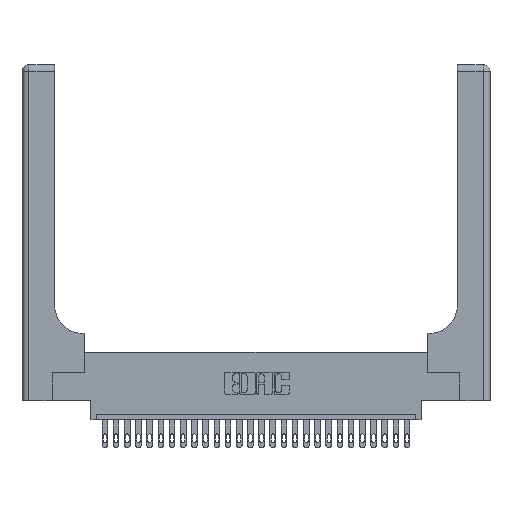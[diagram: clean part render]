
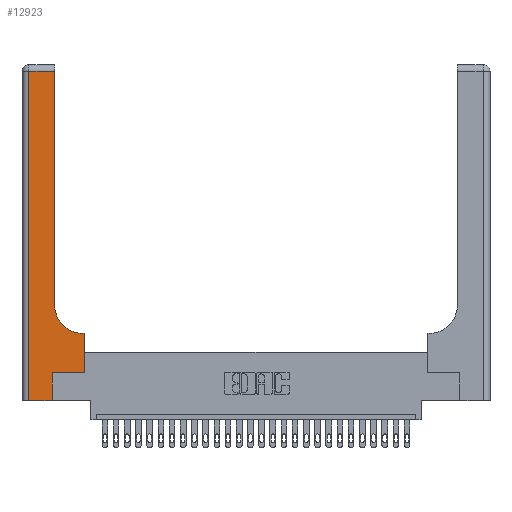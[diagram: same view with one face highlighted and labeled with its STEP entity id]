
A CAD part, top view. The second image highlights one B-rep face of the part: STEP entity #12923.
In plain terms, the highlighted planar face has unit normal (0, 0, 1).
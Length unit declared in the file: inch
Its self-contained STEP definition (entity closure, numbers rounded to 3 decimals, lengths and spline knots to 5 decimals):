
#1087 = VERTEX_POINT ( 'NONE', #15243 ) ;
#1124 = EDGE_CURVE ( 'NONE', #19941, #24948, #12231, .T. ) ;
#1284 = EDGE_CURVE ( 'NONE', #19862, #2779, #8533, .T. ) ;
#1878 = CARTESIAN_POINT ( 'NONE',  ( 0.06, 0., 0.37 ) ) ;
#2245 = CARTESIAN_POINT ( 'NONE',  ( 0.5585, 0.25, 0.37 ) ) ;
#2260 = EDGE_LOOP ( 'NONE', ( #27767, #25125, #16244, #16059, #4777, #15587, #26171, #25153, #7526 ) ) ;
#2608 = EDGE_CURVE ( 'NONE', #4192, #10452, #23671, .T. ) ;
#2779 = VERTEX_POINT ( 'NONE', #12306 ) ;
#2993 = CARTESIAN_POINT ( 'NONE',  ( 0.5415, 0.6, 0.37 ) ) ;
#3927 = CARTESIAN_POINT ( 'NONE',  ( 0.06, 2.94, 0.37 ) ) ;
#4192 = VERTEX_POINT ( 'NONE', #7046 ) ;
#4509 = DIRECTION ( 'NONE',  ( 1., 0., 0. ) ) ;
#4777 = ORIENTED_EDGE ( 'NONE', *, *, #21290, .T. ) ;
#5163 = VECTOR ( 'NONE', #21841, 39.37008 ) ;
#6279 = CARTESIAN_POINT ( 'NONE',  ( 0.2915, 0.85, 0.37 ) ) ;
#6753 = VERTEX_POINT ( 'NONE', #3927 ) ;
#7046 = CARTESIAN_POINT ( 'NONE',  ( 0.5585, 0.6, 0.37 ) ) ;
#7117 = CARTESIAN_POINT ( 'NONE',  ( 0.06, 3., 0.37 ) ) ;
#7526 = ORIENTED_EDGE ( 'NONE', *, *, #10643, .T. ) ;
#8276 = DIRECTION ( 'NONE',  ( -1., 0., 0. ) ) ;
#8343 = CARTESIAN_POINT ( 'NONE',  ( 0., 3., 0.37 ) ) ;
#8533 = LINE ( 'NONE', #26169, #28185 ) ;
#9710 = FACE_OUTER_BOUND ( 'NONE', #2260, .T. ) ;
#10094 = EDGE_CURVE ( 'NONE', #2779, #6753, #20398, .T. ) ;
#10138 = CARTESIAN_POINT ( 'NONE',  ( 0.5585, 0.25, 0.37 ) ) ;
#10452 = VERTEX_POINT ( 'NONE', #2993 ) ;
#10643 = EDGE_CURVE ( 'NONE', #10452, #19862, #11910, .T. ) ;
#10794 = DIRECTION ( 'NONE',  ( 0., 0., -1. ) ) ;
#11910 = CIRCLE ( 'NONE', #17909, 0.25 ) ;
#12019 = EDGE_CURVE ( 'NONE', #24948, #4192, #18613, .T. ) ;
#12231 = LINE ( 'NONE', #18712, #26135 ) ;
#12306 = CARTESIAN_POINT ( 'NONE',  ( 0.2915, 2.94, 0.37 ) ) ;
#12521 = DIRECTION ( 'NONE',  ( 0., 1., 0. ) ) ;
#12923 = ADVANCED_FACE ( 'NONE', ( #9710 ), #27775, .F. ) ;
#12943 = LINE ( 'NONE', #23023, #14644 ) ;
#14063 = AXIS2_PLACEMENT_3D ( 'NONE', #8343, #10794, #14897 ) ;
#14644 = VECTOR ( 'NONE', #16668, 39.37008 ) ;
#14897 = DIRECTION ( 'NONE',  ( -1., 0., 0. ) ) ;
#14948 = CARTESIAN_POINT ( 'NONE',  ( 0.5415, 0.85, 0.37 ) ) ;
#15243 = CARTESIAN_POINT ( 'NONE',  ( 0.269, 0., 0.37 ) ) ;
#15332 = CARTESIAN_POINT ( 'NONE',  ( 0.269, 0., 0.37 ) ) ;
#15587 = ORIENTED_EDGE ( 'NONE', *, *, #1124, .T. ) ;
#16059 = ORIENTED_EDGE ( 'NONE', *, *, #16177, .T. ) ;
#16085 = LINE ( 'NONE', #15332, #5163 ) ;
#16177 = EDGE_CURVE ( 'NONE', #24837, #1087, #12943, .T. ) ;
#16244 = ORIENTED_EDGE ( 'NONE', *, *, #25128, .T. ) ;
#16668 = DIRECTION ( 'NONE',  ( 1., 0., 0. ) ) ;
#17864 = VECTOR ( 'NONE', #22252, 39.37008 ) ;
#17909 = AXIS2_PLACEMENT_3D ( 'NONE', #14948, #28107, #23621 ) ;
#18613 = LINE ( 'NONE', #10138, #21671 ) ;
#18712 = CARTESIAN_POINT ( 'NONE',  ( 0.269, 0.25, 0.37 ) ) ;
#19003 = DIRECTION ( 'NONE',  ( -1., 0., 0. ) ) ;
#19290 = VECTOR ( 'NONE', #19003, 39.37008 ) ;
#19377 = CARTESIAN_POINT ( 'NONE',  ( 0.2915, 0.6, 0.37 ) ) ;
#19862 = VERTEX_POINT ( 'NONE', #6279 ) ;
#19895 = LINE ( 'NONE', #7117, #17864 ) ;
#19941 = VERTEX_POINT ( 'NONE', #27935 ) ;
#20398 = LINE ( 'NONE', #21048, #23800 ) ;
#21048 = CARTESIAN_POINT ( 'NONE',  ( 0., 2.94, 0.37 ) ) ;
#21290 = EDGE_CURVE ( 'NONE', #1087, #19941, #16085, .T. ) ;
#21671 = VECTOR ( 'NONE', #12521, 39.37008 ) ;
#21841 = DIRECTION ( 'NONE',  ( 0., 1., 0. ) ) ;
#22252 = DIRECTION ( 'NONE',  ( 0., -1., 0. ) ) ;
#23023 = CARTESIAN_POINT ( 'NONE',  ( 0., 0., 0.37 ) ) ;
#23621 = DIRECTION ( 'NONE',  ( 1., 0., 0. ) ) ;
#23671 = LINE ( 'NONE', #19377, #19290 ) ;
#23800 = VECTOR ( 'NONE', #8276, 39.37008 ) ;
#24059 = DIRECTION ( 'NONE',  ( 0., 1., 0. ) ) ;
#24837 = VERTEX_POINT ( 'NONE', #1878 ) ;
#24948 = VERTEX_POINT ( 'NONE', #2245 ) ;
#25125 = ORIENTED_EDGE ( 'NONE', *, *, #10094, .T. ) ;
#25128 = EDGE_CURVE ( 'NONE', #6753, #24837, #19895, .T. ) ;
#25153 = ORIENTED_EDGE ( 'NONE', *, *, #2608, .T. ) ;
#26135 = VECTOR ( 'NONE', #4509, 39.37008 ) ;
#26169 = CARTESIAN_POINT ( 'NONE',  ( 0.2915, 3., 0.37 ) ) ;
#26171 = ORIENTED_EDGE ( 'NONE', *, *, #12019, .T. ) ;
#27767 = ORIENTED_EDGE ( 'NONE', *, *, #1284, .T. ) ;
#27775 = PLANE ( 'NONE',  #14063 ) ;
#27935 = CARTESIAN_POINT ( 'NONE',  ( 0.269, 0.25, 0.37 ) ) ;
#28107 = DIRECTION ( 'NONE',  ( 0., 0., -1. ) ) ;
#28185 = VECTOR ( 'NONE', #24059, 39.37008 ) ;
